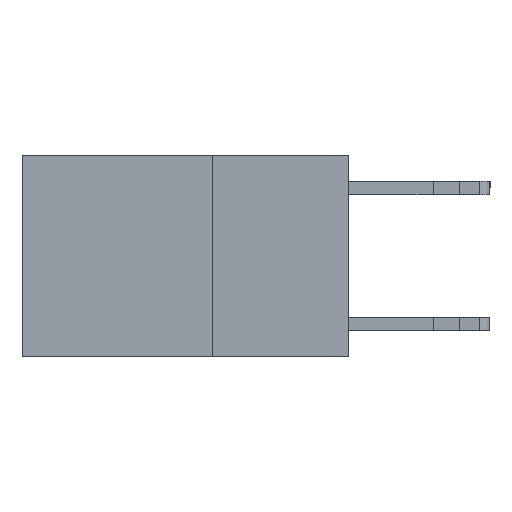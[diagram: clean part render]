
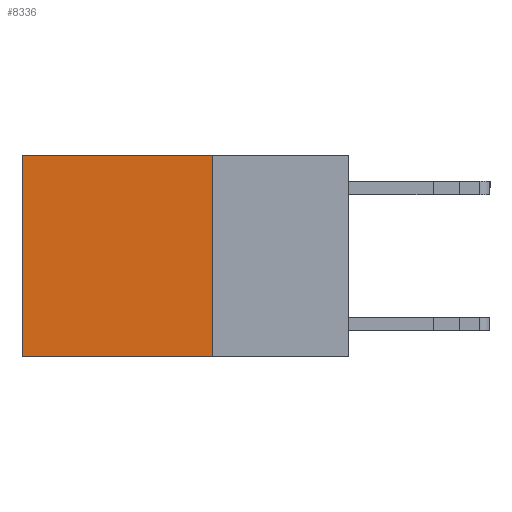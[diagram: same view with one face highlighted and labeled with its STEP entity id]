
A CAD part, left-side view. The second image highlights one B-rep face of the part: STEP entity #8336.
In plain terms, the highlighted planar face has unit normal (-1, 0, 0).
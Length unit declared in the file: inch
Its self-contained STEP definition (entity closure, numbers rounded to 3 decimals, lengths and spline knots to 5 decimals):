
#81 = LINE ( 'NONE', #14064, #13913 ) ;
#1157 = ORIENTED_EDGE ( 'NONE', *, *, #4169, .F. ) ;
#2118 = CARTESIAN_POINT ( 'NONE',  ( 0.2625, 0.25, -0.37 ) ) ;
#2583 = CARTESIAN_POINT ( 'NONE',  ( 0.2625, 0.25, 0. ) ) ;
#3208 = ORIENTED_EDGE ( 'NONE', *, *, #8752, .T. ) ;
#3327 = ORIENTED_EDGE ( 'NONE', *, *, #11928, .F. ) ;
#3452 = EDGE_LOOP ( 'NONE', ( #3208, #1157, #3327, #12287 ) ) ;
#4026 = CARTESIAN_POINT ( 'NONE',  ( 0.2625, 0.25, -0.37 ) ) ;
#4169 = EDGE_CURVE ( 'NONE', #9803, #11931, #11522, .T. ) ;
#5203 = VERTEX_POINT ( 'NONE', #13812 ) ;
#5966 = CARTESIAN_POINT ( 'NONE',  ( 0.2625, 0.6, -0.37 ) ) ;
#6277 = EDGE_CURVE ( 'NONE', #6349, #5203, #7499, .T. ) ;
#6349 = VERTEX_POINT ( 'NONE', #9823 ) ;
#6661 = LINE ( 'NONE', #7802, #7247 ) ;
#7212 = DIRECTION ( 'NONE',  ( 1., 0., 0. ) ) ;
#7247 = VECTOR ( 'NONE', #12478, 39.37008 ) ;
#7499 = LINE ( 'NONE', #13175, #8954 ) ;
#7582 = AXIS2_PLACEMENT_3D ( 'NONE', #2583, #7212, #13107 ) ;
#7802 = CARTESIAN_POINT ( 'NONE',  ( 0.2625, 0.6, 0. ) ) ;
#8336 = ADVANCED_FACE ( 'NONE', ( #12883 ), #9532, .F. ) ;
#8752 = EDGE_CURVE ( 'NONE', #5203, #11931, #6661, .T. ) ;
#8904 = DIRECTION ( 'NONE',  ( 0., 1., 0. ) ) ;
#8954 = VECTOR ( 'NONE', #9894, 39.37008 ) ;
#9532 = PLANE ( 'NONE',  #7582 ) ;
#9803 = VERTEX_POINT ( 'NONE', #4026 ) ;
#9823 = CARTESIAN_POINT ( 'NONE',  ( 0.2625, 0.25, 0. ) ) ;
#9894 = DIRECTION ( 'NONE',  ( 0., 1., 0. ) ) ;
#11522 = LINE ( 'NONE', #2118, #14645 ) ;
#11798 = DIRECTION ( 'NONE',  ( 0., 0., -1. ) ) ;
#11928 = EDGE_CURVE ( 'NONE', #6349, #9803, #81, .T. ) ;
#11931 = VERTEX_POINT ( 'NONE', #5966 ) ;
#12287 = ORIENTED_EDGE ( 'NONE', *, *, #6277, .T. ) ;
#12478 = DIRECTION ( 'NONE',  ( 0., 0., -1. ) ) ;
#12883 = FACE_OUTER_BOUND ( 'NONE', #3452, .T. ) ;
#13107 = DIRECTION ( 'NONE',  ( 0., 0., -1. ) ) ;
#13175 = CARTESIAN_POINT ( 'NONE',  ( 0.2625, 0.25, 0. ) ) ;
#13812 = CARTESIAN_POINT ( 'NONE',  ( 0.2625, 0.6, 0. ) ) ;
#13913 = VECTOR ( 'NONE', #11798, 39.37008 ) ;
#14064 = CARTESIAN_POINT ( 'NONE',  ( 0.2625, 0.25, 0. ) ) ;
#14645 = VECTOR ( 'NONE', #8904, 39.37008 ) ;
